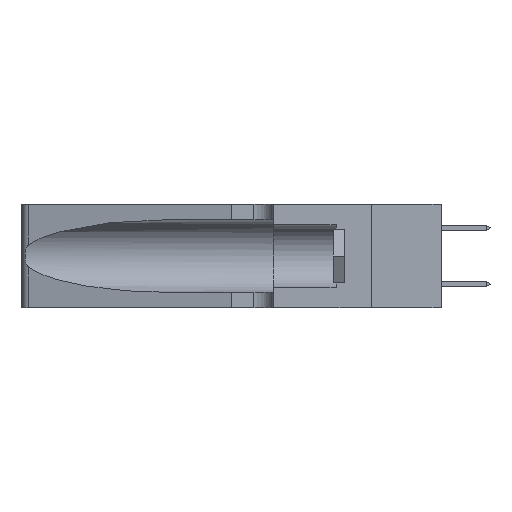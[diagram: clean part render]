
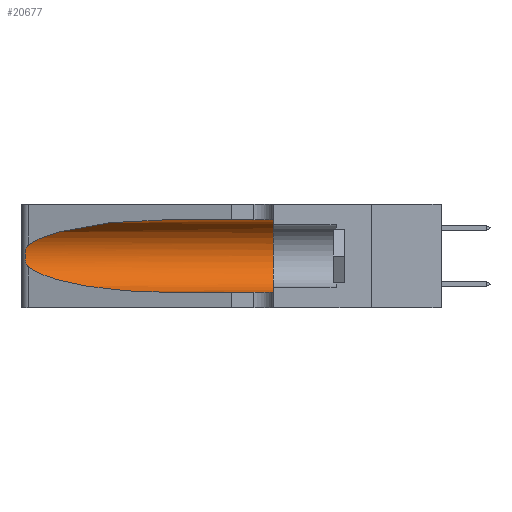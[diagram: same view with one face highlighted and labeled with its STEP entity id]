
A CAD part, left-side view. The second image highlights one B-rep face of the part: STEP entity #20677.
In plain terms, the highlighted cylindrical face has radius 3.308 mm (diameter 6.617 mm), a partial arc.
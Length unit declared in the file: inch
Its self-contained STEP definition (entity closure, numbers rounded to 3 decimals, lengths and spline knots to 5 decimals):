
#221 = EDGE_CURVE ( 'NONE', #5439, #21945, #1145, .T. ) ;
#540 = CARTESIAN_POINT ( 'NONE',  ( 0.18966, 0.96281, 0.31525 ) ) ;
#1145 = LINE ( 'NONE', #23684, #19433 ) ;
#1777 = CARTESIAN_POINT ( 'NONE',  ( 0.25854, 1.2359, 0.20912 ) ) ;
#1861 = ORIENTED_EDGE ( 'NONE', *, *, #11610, .F. ) ;
#2946 = DIRECTION ( 'NONE',  ( 0., -1., 0. ) ) ;
#4170 = CARTESIAN_POINT ( 'NONE',  ( 0.26075, 1.23896, 0.19203 ) ) ;
#4810 = ORIENTED_EDGE ( 'NONE', *, *, #27803, .F. ) ;
#5136 = FACE_OUTER_BOUND ( 'NONE', #22698, .T. ) ;
#5272 = DIRECTION ( 'NONE',  ( 0., -1., 0. ) ) ;
#5345 = CARTESIAN_POINT ( 'NONE',  ( 0.2373, 1.15595, 0.28018 ) ) ;
#5439 = VERTEX_POINT ( 'NONE', #25165 ) ;
#5572 = CARTESIAN_POINT ( 'NONE',  ( 0.1305, 0.35, 0.31525 ) ) ;
#5989 = EDGE_CURVE ( 'NONE', #18744, #8874, #7273, .T. ) ;
#6583 = CARTESIAN_POINT ( 'NONE',  ( 0.26017, 1.23833, 0.17102 ) ) ;
#6888 = DIRECTION ( 'NONE',  ( 0., 1., 0. ) ) ;
#7273 = B_SPLINE_CURVE_WITH_KNOTS ( 'NONE', 3,
 ( #11274, #13703, #27825, #16095, #1777, #18467, #4170, #20834, #6583, #23181, #8989, #25558, #11379, #27923 ),
 .UNSPECIFIED., .F., .F.,
 ( 4, 2, 2, 2, 2, 2, 4 ),
 ( 0., 0.00027, 0.00053, 0.00107, 0.0016, 0.00187, 0.00214 ),
 .UNSPECIFIED. ) ;
#8148 = DIRECTION ( 'NONE',  ( 0., -1., 0. ) ) ;
#8395 = CARTESIAN_POINT ( 'NONE',  ( 0.1305, 0.72297, 0.31525 ) ) ;
#8778 = CIRCLE ( 'NONE', #15923, 0.13025 ) ;
#8874 = VERTEX_POINT ( 'NONE', #14382 ) ;
#8989 = CARTESIAN_POINT ( 'NONE',  ( 0.25789, 1.23486, 0.15765 ) ) ;
#11274 = CARTESIAN_POINT ( 'NONE',  ( 0.25487, 1.22718, 0.22369 ) ) ;
#11379 = CARTESIAN_POINT ( 'NONE',  ( 0.25555, 1.22993, 0.14849 ) ) ;
#11610 = EDGE_CURVE ( 'NONE', #28796, #18008, #15159, .T. ) ;
#12856 = CARTESIAN_POINT ( 'NONE',  ( 0.1305, 1.61858, 0.185 ) ) ;
#13421 = ORIENTED_EDGE ( 'NONE', *, *, #221, .T. ) ;
#13703 = CARTESIAN_POINT ( 'NONE',  ( 0.25555, 1.22994, 0.2215 ) ) ;
#14304 = CARTESIAN_POINT ( 'NONE',  ( 0.1305, 0.72297, 0.05475 ) ) ;
#14382 = CARTESIAN_POINT ( 'NONE',  ( 0.25487, 1.22718, 0.14631 ) ) ;
#15159 = LINE ( 'NONE', #21961, #20688 ) ;
#15923 = AXIS2_PLACEMENT_3D ( 'NONE', #21132, #6888, #23471 ) ;
#16095 = CARTESIAN_POINT ( 'NONE',  ( 0.25787, 1.23484, 0.2124 ) ) ;
#17243 = CARTESIAN_POINT ( 'NONE',  ( 0.1305, 0.72297, 0.31525 ) ) ;
#17527 = CARTESIAN_POINT ( 'NONE',  ( 0.25487, 1.22718, 0.22369 ) ) ;
#17718 = ORIENTED_EDGE ( 'NONE', *, *, #5989, .T. ) ;
#18008 = VERTEX_POINT ( 'NONE', #5572 ) ;
#18467 = CARTESIAN_POINT ( 'NONE',  ( 0.26018, 1.23835, 0.19895 ) ) ;
#18744 = VERTEX_POINT ( 'NONE', #17527 ) ;
#19117 = EDGE_CURVE ( 'NONE', #8874, #5439, #29013, .T. ) ;
#19433 = VECTOR ( 'NONE', #5272, 39.37008 ) ;
#20677 = ADVANCED_FACE ( 'NONE', ( #5136 ), #23339, .F. ) ;
#20688 = VECTOR ( 'NONE', #2946, 39.37008 ) ;
#20834 = CARTESIAN_POINT ( 'NONE',  ( 0.26075, 1.23896, 0.178 ) ) ;
#21132 = CARTESIAN_POINT ( 'NONE',  ( 0.1305, 0.35, 0.185 ) ) ;
#21319 = CARTESIAN_POINT ( 'NONE',  ( 0.25487, 1.22718, 0.14631 ) ) ;
#21753 =( BOUNDED_CURVE ( )  B_SPLINE_CURVE ( 3, ( #17243, #540, #5345, #21966 ),
 .UNSPECIFIED., .F., .F. ) 
 B_SPLINE_CURVE_WITH_KNOTS ( ( 4, 4 ),
 ( 1.5708, 2.84003 ),
 .UNSPECIFIED. ) 
 CURVE ( )  GEOMETRIC_REPRESENTATION_ITEM ( )  RATIONAL_B_SPLINE_CURVE ( ( 1., 0.87, 0.87, 1. ) ) 
 REPRESENTATION_ITEM ( '' )  );
#21945 = VERTEX_POINT ( 'NONE', #26873 ) ;
#21961 = CARTESIAN_POINT ( 'NONE',  ( 0.1305, 1.61858, 0.31525 ) ) ;
#21966 = CARTESIAN_POINT ( 'NONE',  ( 0.25487, 1.22718, 0.22369 ) ) ;
#22698 = EDGE_LOOP ( 'NONE', ( #27983, #17718, #23050, #13421, #4810, #1861 ) ) ;
#23050 = ORIENTED_EDGE ( 'NONE', *, *, #19117, .T. ) ;
#23181 = CARTESIAN_POINT ( 'NONE',  ( 0.25856, 1.23593, 0.16098 ) ) ;
#23305 = EDGE_CURVE ( 'NONE', #28796, #18744, #21753, .T. ) ;
#23339 = CYLINDRICAL_SURFACE ( 'NONE', #27238, 0.13025 ) ;
#23471 = DIRECTION ( 'NONE',  ( 0., 0., 1. ) ) ;
#23684 = CARTESIAN_POINT ( 'NONE',  ( 0.1305, 1.61858, 0.05475 ) ) ;
#24731 = DIRECTION ( 'NONE',  ( 0., 0., -1. ) ) ;
#25165 = CARTESIAN_POINT ( 'NONE',  ( 0.1305, 0.72297, 0.05475 ) ) ;
#25558 = CARTESIAN_POINT ( 'NONE',  ( 0.25639, 1.23186, 0.15144 ) ) ;
#26042 = CARTESIAN_POINT ( 'NONE',  ( 0.2373, 1.15595, 0.08982 ) ) ;
#26873 = CARTESIAN_POINT ( 'NONE',  ( 0.1305, 0.35, 0.05475 ) ) ;
#27238 = AXIS2_PLACEMENT_3D ( 'NONE', #12856, #8148, #24731 ) ;
#27803 = EDGE_CURVE ( 'NONE', #18008, #21945, #8778, .T. ) ;
#27825 = CARTESIAN_POINT ( 'NONE',  ( 0.25639, 1.23184, 0.21858 ) ) ;
#27923 = CARTESIAN_POINT ( 'NONE',  ( 0.25487, 1.22718, 0.14631 ) ) ;
#27983 = ORIENTED_EDGE ( 'NONE', *, *, #23305, .T. ) ;
#28414 = CARTESIAN_POINT ( 'NONE',  ( 0.18966, 0.96281, 0.05475 ) ) ;
#28796 = VERTEX_POINT ( 'NONE', #8395 ) ;
#29013 =( BOUNDED_CURVE ( )  B_SPLINE_CURVE ( 3, ( #21319, #26042, #28414, #14304 ),
 .UNSPECIFIED., .F., .F. ) 
 B_SPLINE_CURVE_WITH_KNOTS ( ( 4, 4 ),
 ( 3.44316, 4.71239 ),
 .UNSPECIFIED. ) 
 CURVE ( )  GEOMETRIC_REPRESENTATION_ITEM ( )  RATIONAL_B_SPLINE_CURVE ( ( 1., 0.87, 0.87, 1. ) ) 
 REPRESENTATION_ITEM ( '' )  );
